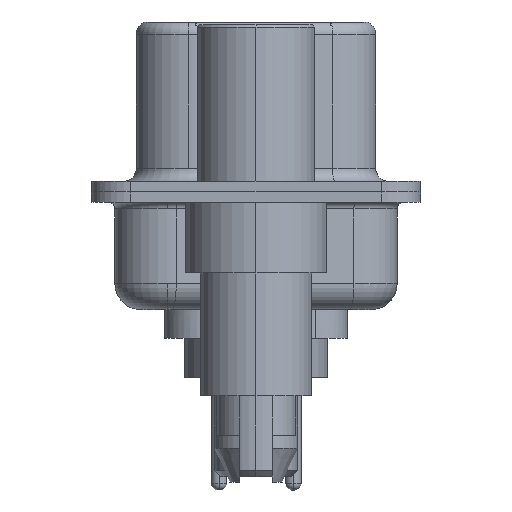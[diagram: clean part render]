
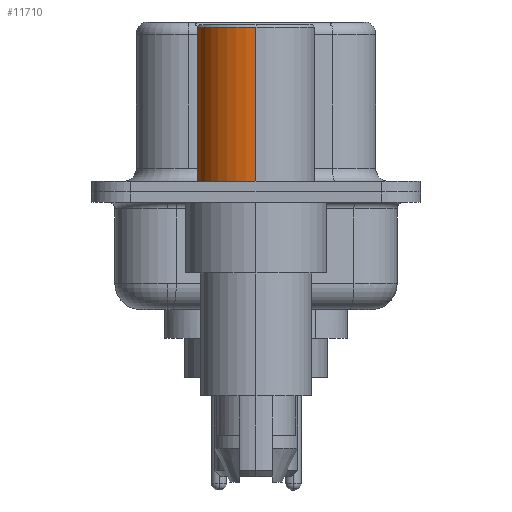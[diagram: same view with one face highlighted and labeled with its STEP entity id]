
A CAD part, left-side view. The second image highlights one B-rep face of the part: STEP entity #11710.
In plain terms, the highlighted cylindrical face has radius 2.25 mm (diameter 4.5 mm), a partial arc.
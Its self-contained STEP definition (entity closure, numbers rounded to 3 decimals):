
#166 = EDGE_CURVE ( 'NONE', #7535, #5335, #14305, .T. ) ;
#213 = VERTEX_POINT ( 'NONE', #13954 ) ;
#932 = CARTESIAN_POINT ( 'NONE',  ( 2.25, 0., 0.581 ) ) ;
#1511 = EDGE_LOOP ( 'NONE', ( #9959, #17533, #15248, #8098 ) ) ;
#2623 = EDGE_CURVE ( 'NONE', #213, #11748, #16085, .T. ) ;
#2799 = AXIS2_PLACEMENT_3D ( 'NONE', #8258, #4232, #20721 ) ;
#3076 = DIRECTION ( 'NONE',  ( 0., 0., 1. ) ) ;
#4232 = DIRECTION ( 'NONE',  ( 0., 0., 1. ) ) ;
#5087 = DIRECTION ( 'NONE',  ( 0., 0., 1. ) ) ;
#5158 = LINE ( 'NONE', #22085, #14914 ) ;
#5335 = VERTEX_POINT ( 'NONE', #17824 ) ;
#5708 = CARTESIAN_POINT ( 'NONE',  ( 0., 0., 0.4 ) ) ;
#7535 = VERTEX_POINT ( 'NONE', #18108 ) ;
#8098 = ORIENTED_EDGE ( 'NONE', *, *, #16206, .F. ) ;
#8258 = CARTESIAN_POINT ( 'NONE',  ( 0., 0., 0.581 ) ) ;
#8535 = CARTESIAN_POINT ( 'NONE',  ( -2.25, 0., 6.3 ) ) ;
#9959 = ORIENTED_EDGE ( 'NONE', *, *, #166, .T. ) ;
#10827 = CARTESIAN_POINT ( 'NONE',  ( 0., 0., 6.3 ) ) ;
#10921 = DIRECTION ( 'NONE',  ( 0., 0., 1. ) ) ;
#11566 = FACE_OUTER_BOUND ( 'NONE', #1511, .T. ) ;
#11710 = ADVANCED_FACE ( 'NONE', ( #11566 ), #16415, .T. ) ;
#11748 = VERTEX_POINT ( 'NONE', #8535 ) ;
#12206 = AXIS2_PLACEMENT_3D ( 'NONE', #10827, #10921, #18200 ) ;
#13910 = DIRECTION ( 'NONE',  ( 0., 0., 1. ) ) ;
#13954 = CARTESIAN_POINT ( 'NONE',  ( 2.25, 0., 6.3 ) ) ;
#14305 = CIRCLE ( 'NONE', #21443, 2.25 ) ;
#14914 = VECTOR ( 'NONE', #13910, 1000. ) ;
#15123 = DIRECTION ( 'NONE',  ( 1., 0., 0. ) ) ;
#15248 = ORIENTED_EDGE ( 'NONE', *, *, #2623, .F. ) ;
#16085 = CIRCLE ( 'NONE', #12206, 2.25 ) ;
#16206 = EDGE_CURVE ( 'NONE', #7535, #213, #19370, .T. ) ;
#16415 = CYLINDRICAL_SURFACE ( 'NONE', #2799, 2.25 ) ;
#17533 = ORIENTED_EDGE ( 'NONE', *, *, #21203, .T. ) ;
#17824 = CARTESIAN_POINT ( 'NONE',  ( -2.25, 0., 0.4 ) ) ;
#18108 = CARTESIAN_POINT ( 'NONE',  ( 2.25, 0., 0.4 ) ) ;
#18200 = DIRECTION ( 'NONE',  ( 1., 0., 0. ) ) ;
#19370 = LINE ( 'NONE', #932, #25034 ) ;
#20721 = DIRECTION ( 'NONE',  ( 1., 0., 0. ) ) ;
#21203 = EDGE_CURVE ( 'NONE', #5335, #11748, #5158, .T. ) ;
#21443 = AXIS2_PLACEMENT_3D ( 'NONE', #5708, #5087, #15123 ) ;
#22085 = CARTESIAN_POINT ( 'NONE',  ( -2.25, 0., 0.581 ) ) ;
#25034 = VECTOR ( 'NONE', #3076, 1000. ) ;
